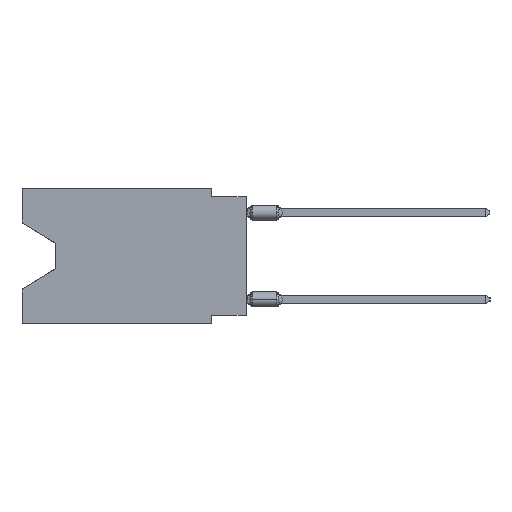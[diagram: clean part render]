
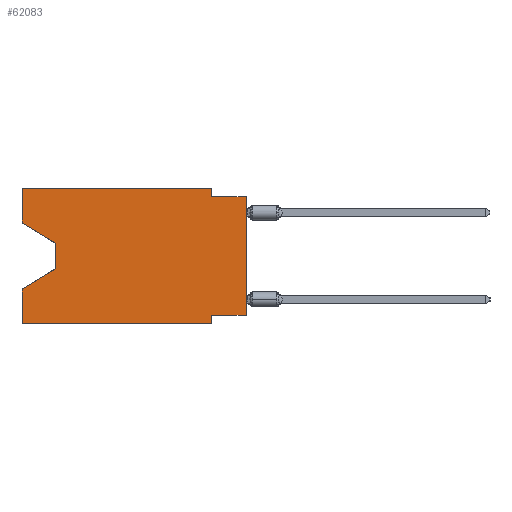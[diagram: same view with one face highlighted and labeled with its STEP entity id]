
A CAD part, left-side view. The second image highlights one B-rep face of the part: STEP entity #62083.
In plain terms, the highlighted planar face has unit normal (-1, 0, 0).
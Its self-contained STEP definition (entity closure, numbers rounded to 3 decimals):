
#402 = ORIENTED_EDGE ( 'NONE', *, *, #4937, .T. ) ;
#502 = VERTEX_POINT ( 'NONE', #5838 ) ;
#1007 = DIRECTION ( 'NONE',  ( 0., 0., 1. ) ) ;
#1167 = CARTESIAN_POINT ( 'NONE',  ( 0., 0., -0.635 ) ) ;
#1401 = VERTEX_POINT ( 'NONE', #56615 ) ;
#1800 = CARTESIAN_POINT ( 'NONE',  ( 0., 16.383, 0. ) ) ;
#1838 = EDGE_CURVE ( 'NONE', #49842, #502, #3436, .T. ) ;
#2096 = CARTESIAN_POINT ( 'NONE',  ( 0., 13.97, -5.893 ) ) ;
#3436 = LINE ( 'NONE', #29224, #30379 ) ;
#4371 = VERTEX_POINT ( 'NONE', #24642 ) ;
#4937 = EDGE_CURVE ( 'NONE', #49842, #37922, #40278, .T. ) ;
#5113 = VERTEX_POINT ( 'NONE', #34434 ) ;
#5838 = CARTESIAN_POINT ( 'NONE',  ( 0., 2.54, -9.271 ) ) ;
#6205 = VECTOR ( 'NONE', #21971, 1000. ) ;
#6842 = CARTESIAN_POINT ( 'NONE',  ( 0., 16.383, 0. ) ) ;
#9058 = CARTESIAN_POINT ( 'NONE',  ( 0., 13.97, -4.013 ) ) ;
#10815 = DIRECTION ( 'NONE',  ( 0., 0., -1. ) ) ;
#11339 = CARTESIAN_POINT ( 'NONE',  ( 0., 16.383, -9.906 ) ) ;
#11460 = VECTOR ( 'NONE', #22068, 1000. ) ;
#11857 = DIRECTION ( 'NONE',  ( 1., 0., 0. ) ) ;
#12208 = DIRECTION ( 'NONE',  ( 0., -1., 0. ) ) ;
#12864 = ORIENTED_EDGE ( 'NONE', *, *, #40920, .F. ) ;
#13342 = CARTESIAN_POINT ( 'NONE',  ( 0., 16.383, 0. ) ) ;
#14254 = ORIENTED_EDGE ( 'NONE', *, *, #50215, .F. ) ;
#14893 = DIRECTION ( 'NONE',  ( 0., 0., -1. ) ) ;
#17041 = CARTESIAN_POINT ( 'NONE',  ( 0., 16.383, 0. ) ) ;
#17579 = VERTEX_POINT ( 'NONE', #26257 ) ;
#18538 = VERTEX_POINT ( 'NONE', #24596 ) ;
#18928 = CARTESIAN_POINT ( 'NONE',  ( 0., 16.383, -2.546 ) ) ;
#21116 = CARTESIAN_POINT ( 'NONE',  ( 0., 0., 0. ) ) ;
#21430 = EDGE_CURVE ( 'NONE', #18538, #5113, #27757, .T. ) ;
#21920 = EDGE_CURVE ( 'NONE', #18538, #38391, #49414, .T. ) ;
#21971 = DIRECTION ( 'NONE',  ( 0., 0., -1. ) ) ;
#22068 = DIRECTION ( 'NONE',  ( 0., -1., 0. ) ) ;
#22255 = PLANE ( 'NONE',  #30665 ) ;
#22258 = CARTESIAN_POINT ( 'NONE',  ( 0., 2.54, -0.635 ) ) ;
#22554 = VECTOR ( 'NONE', #10815, 1000. ) ;
#22720 = DIRECTION ( 'NONE',  ( 0., 0., 1. ) ) ;
#23187 = EDGE_CURVE ( 'NONE', #38391, #1401, #55120, .T. ) ;
#23309 = VERTEX_POINT ( 'NONE', #22258 ) ;
#24596 = CARTESIAN_POINT ( 'NONE',  ( 0., 16.383, -2.546 ) ) ;
#24642 = CARTESIAN_POINT ( 'NONE',  ( 0., 2.54, 0. ) ) ;
#26257 = CARTESIAN_POINT ( 'NONE',  ( 0., 16.383, -9.906 ) ) ;
#27141 = VERTEX_POINT ( 'NONE', #35795 ) ;
#27513 = ORIENTED_EDGE ( 'NONE', *, *, #43811, .F. ) ;
#27757 = LINE ( 'NONE', #17041, #50132 ) ;
#28944 = ORIENTED_EDGE ( 'NONE', *, *, #21430, .F. ) ;
#29224 = CARTESIAN_POINT ( 'NONE',  ( 0., 0., -9.271 ) ) ;
#29535 = DIRECTION ( 'NONE',  ( 0., -1., 0. ) ) ;
#30379 = VECTOR ( 'NONE', #43646, 1000. ) ;
#30665 = AXIS2_PLACEMENT_3D ( 'NONE', #1800, #11857, #52403 ) ;
#31125 = VECTOR ( 'NONE', #58911, 1000. ) ;
#32019 = EDGE_CURVE ( 'NONE', #17579, #27141, #58230, .T. ) ;
#34434 = CARTESIAN_POINT ( 'NONE',  ( 0., 16.383, 0. ) ) ;
#35433 = ORIENTED_EDGE ( 'NONE', *, *, #48853, .T. ) ;
#35459 = ORIENTED_EDGE ( 'NONE', *, *, #21920, .T. ) ;
#35795 = CARTESIAN_POINT ( 'NONE',  ( 0., 2.54, -9.906 ) ) ;
#37922 = VERTEX_POINT ( 'NONE', #1167 ) ;
#37930 = EDGE_CURVE ( 'NONE', #5113, #4371, #52759, .T. ) ;
#38156 = ORIENTED_EDGE ( 'NONE', *, *, #23187, .T. ) ;
#38391 = VERTEX_POINT ( 'NONE', #9058 ) ;
#38473 = LINE ( 'NONE', #13342, #31125 ) ;
#39022 = CARTESIAN_POINT ( 'NONE',  ( 0., 0., -9.271 ) ) ;
#39349 = DIRECTION ( 'NONE',  ( 0., -0.855, -0.519 ) ) ;
#39542 = ORIENTED_EDGE ( 'NONE', *, *, #37930, .F. ) ;
#40278 = LINE ( 'NONE', #21116, #42551 ) ;
#40920 = EDGE_CURVE ( 'NONE', #502, #27141, #57807, .T. ) ;
#41644 = CARTESIAN_POINT ( 'NONE',  ( 0., 2.54, 0. ) ) ;
#42011 = VERTEX_POINT ( 'NONE', #54919 ) ;
#42551 = VECTOR ( 'NONE', #1007, 1000. ) ;
#42639 = LINE ( 'NONE', #2096, #65791 ) ;
#43033 = CARTESIAN_POINT ( 'NONE',  ( 0., 2.54, -9.906 ) ) ;
#43646 = DIRECTION ( 'NONE',  ( 0., 1., 0. ) ) ;
#43811 = EDGE_CURVE ( 'NONE', #4371, #23309, #58053, .T. ) ;
#47058 = VECTOR ( 'NONE', #14893, 1000. ) ;
#47681 = VECTOR ( 'NONE', #29535, 1000. ) ;
#48853 = EDGE_CURVE ( 'NONE', #1401, #42011, #42639, .T. ) ;
#49009 = CARTESIAN_POINT ( 'NONE',  ( 0., 0., -0.635 ) ) ;
#49414 = LINE ( 'NONE', #18928, #64075 ) ;
#49842 = VERTEX_POINT ( 'NONE', #39022 ) ;
#50132 = VECTOR ( 'NONE', #22720, 1000. ) ;
#50215 = EDGE_CURVE ( 'NONE', #23309, #37922, #54687, .T. ) ;
#52403 = DIRECTION ( 'NONE',  ( 0., 0., -1. ) ) ;
#52759 = LINE ( 'NONE', #6842, #53188 ) ;
#53188 = VECTOR ( 'NONE', #12208, 1000. ) ;
#53585 = ORIENTED_EDGE ( 'NONE', *, *, #32019, .T. ) ;
#54687 = LINE ( 'NONE', #49009, #47681 ) ;
#54919 = CARTESIAN_POINT ( 'NONE',  ( 0., 16.383, -7.36 ) ) ;
#55120 = LINE ( 'NONE', #60130, #47058 ) ;
#56615 = CARTESIAN_POINT ( 'NONE',  ( 0., 13.97, -5.893 ) ) ;
#57037 = ORIENTED_EDGE ( 'NONE', *, *, #64712, .F. ) ;
#57668 = EDGE_LOOP ( 'NONE', ( #35459, #38156, #35433, #57037, #53585, #12864, #65593, #402, #14254, #27513, #39542, #28944 ) ) ;
#57807 = LINE ( 'NONE', #43033, #6205 ) ;
#58053 = LINE ( 'NONE', #41644, #22554 ) ;
#58230 = LINE ( 'NONE', #11339, #11460 ) ;
#58911 = DIRECTION ( 'NONE',  ( 0., 0., 1. ) ) ;
#60130 = CARTESIAN_POINT ( 'NONE',  ( 0., 13.97, -4.013 ) ) ;
#62083 = ADVANCED_FACE ( 'NONE', ( #63106 ), #22255, .F. ) ;
#63078 = DIRECTION ( 'NONE',  ( 0., 0.855, -0.519 ) ) ;
#63106 = FACE_OUTER_BOUND ( 'NONE', #57668, .T. ) ;
#64075 = VECTOR ( 'NONE', #39349, 1000. ) ;
#64712 = EDGE_CURVE ( 'NONE', #17579, #42011, #38473, .T. ) ;
#65593 = ORIENTED_EDGE ( 'NONE', *, *, #1838, .F. ) ;
#65791 = VECTOR ( 'NONE', #63078, 1000. ) ;
